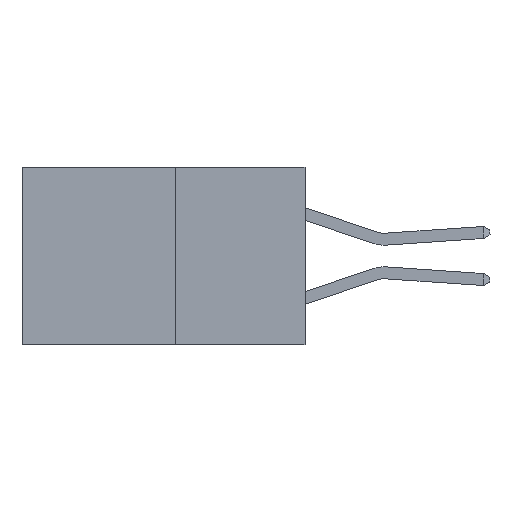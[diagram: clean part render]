
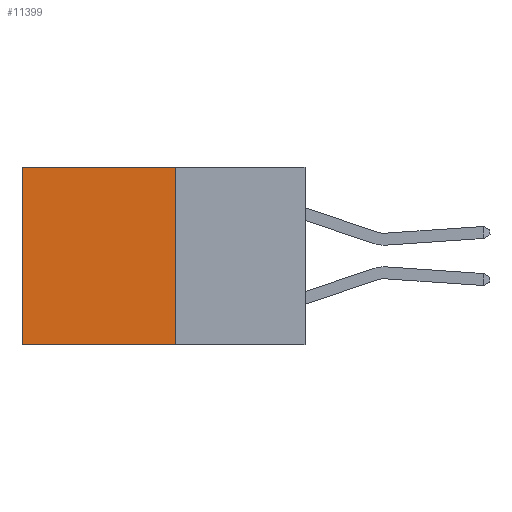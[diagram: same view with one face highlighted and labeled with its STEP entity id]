
A CAD part, left-side view. The second image highlights one B-rep face of the part: STEP entity #11399.
In plain terms, the highlighted planar face has unit normal (-1, 0, 0).
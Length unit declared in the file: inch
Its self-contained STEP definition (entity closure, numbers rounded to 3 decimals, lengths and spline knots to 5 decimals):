
#550 = CARTESIAN_POINT ( 'NONE',  ( 0.277, 0.27, 0. ) ) ;
#2362 = AXIS2_PLACEMENT_3D ( 'NONE', #7973, #12895, #3106 ) ;
#3039 = PLANE ( 'NONE',  #2362 ) ;
#3106 = DIRECTION ( 'NONE',  ( 0., 0., -1. ) ) ;
#4591 = DIRECTION ( 'NONE',  ( 0., 1., 0. ) ) ;
#4601 = CARTESIAN_POINT ( 'NONE',  ( 0.277, 0.59, -0.37 ) ) ;
#5788 = CARTESIAN_POINT ( 'NONE',  ( 0.277, 0.27, -0.37 ) ) ;
#5986 = ORIENTED_EDGE ( 'NONE', *, *, #16634, .F. ) ;
#6114 = VERTEX_POINT ( 'NONE', #20047 ) ;
#6781 = VERTEX_POINT ( 'NONE', #12888 ) ;
#6837 = VECTOR ( 'NONE', #4591, 39.37008 ) ;
#7973 = CARTESIAN_POINT ( 'NONE',  ( 0.277, 0.27, -0.37 ) ) ;
#8151 = LINE ( 'NONE', #4601, #15967 ) ;
#9603 = DIRECTION ( 'NONE',  ( 0., 0., -1. ) ) ;
#10026 = VERTEX_POINT ( 'NONE', #550 ) ;
#10625 = LINE ( 'NONE', #14510, #6837 ) ;
#11399 = ADVANCED_FACE ( 'NONE', ( #14651 ), #3039, .F. ) ;
#12320 = CARTESIAN_POINT ( 'NONE',  ( 0.277, 0.27, -0.37 ) ) ;
#12322 = ORIENTED_EDGE ( 'NONE', *, *, #15726, .T. ) ;
#12888 = CARTESIAN_POINT ( 'NONE',  ( 0.277, 0.59, -0.37 ) ) ;
#12895 = DIRECTION ( 'NONE',  ( 1., 0., 0. ) ) ;
#12977 = VECTOR ( 'NONE', #17408, 39.37008 ) ;
#13006 = EDGE_CURVE ( 'NONE', #10026, #6114, #10625, .T. ) ;
#13849 = VERTEX_POINT ( 'NONE', #19795 ) ;
#14012 = DIRECTION ( 'NONE',  ( 0., 0., -1. ) ) ;
#14510 = CARTESIAN_POINT ( 'NONE',  ( 0.277, 0.27, 0. ) ) ;
#14651 = FACE_OUTER_BOUND ( 'NONE', #16163, .T. ) ;
#14847 = EDGE_CURVE ( 'NONE', #10026, #13849, #16003, .T. ) ;
#15100 = ORIENTED_EDGE ( 'NONE', *, *, #13006, .T. ) ;
#15726 = EDGE_CURVE ( 'NONE', #6114, #6781, #8151, .T. ) ;
#15967 = VECTOR ( 'NONE', #9603, 39.37008 ) ;
#16003 = LINE ( 'NONE', #5788, #19878 ) ;
#16163 = EDGE_LOOP ( 'NONE', ( #12322, #5986, #19150, #15100 ) ) ;
#16634 = EDGE_CURVE ( 'NONE', #13849, #6781, #17991, .T. ) ;
#17408 = DIRECTION ( 'NONE',  ( 0., 1., 0. ) ) ;
#17991 = LINE ( 'NONE', #12320, #12977 ) ;
#19150 = ORIENTED_EDGE ( 'NONE', *, *, #14847, .F. ) ;
#19795 = CARTESIAN_POINT ( 'NONE',  ( 0.277, 0.27, -0.37 ) ) ;
#19878 = VECTOR ( 'NONE', #14012, 39.37008 ) ;
#20047 = CARTESIAN_POINT ( 'NONE',  ( 0.277, 0.59, 0. ) ) ;
